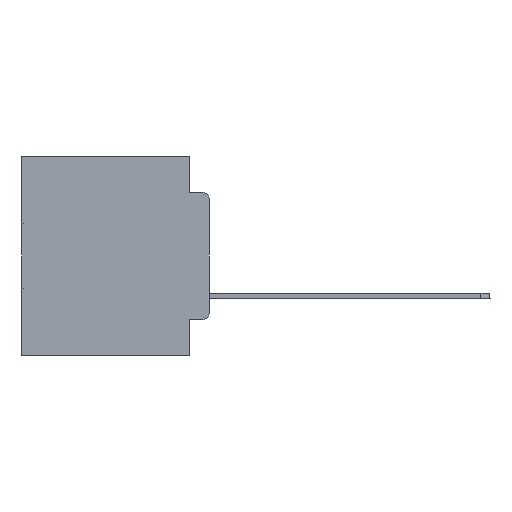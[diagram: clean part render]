
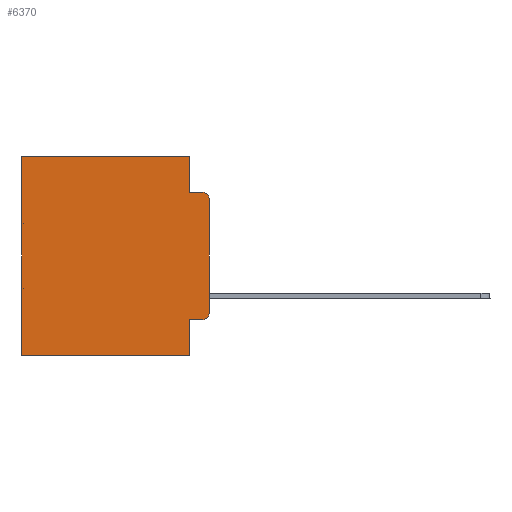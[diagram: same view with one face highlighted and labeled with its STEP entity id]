
A CAD part, left-side view. The second image highlights one B-rep face of the part: STEP entity #6370.
In plain terms, the highlighted planar face has unit normal (-1, 0, 0).
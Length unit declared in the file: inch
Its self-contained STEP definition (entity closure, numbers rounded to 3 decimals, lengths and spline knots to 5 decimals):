
#799 = EDGE_CURVE ( 'NONE', #15589, #9486, #19272, .T. ) ;
#1343 = CARTESIAN_POINT ( 'NONE',  ( 0.298, 0.473, 0. ) ) ;
#1909 = VERTEX_POINT ( 'NONE', #21501 ) ;
#2618 = CARTESIAN_POINT ( 'NONE',  ( 0.298, 0.051, -0.4115 ) ) ;
#3227 = PLANE ( 'NONE',  #21137 ) ;
#3861 = VERTEX_POINT ( 'NONE', #28291 ) ;
#4021 = EDGE_CURVE ( 'NONE', #1909, #19858, #5261, .T. ) ;
#4285 = DIRECTION ( 'NONE',  ( 0., 0., -1. ) ) ;
#5261 = LINE ( 'NONE', #8341, #31345 ) ;
#5583 = ORIENTED_EDGE ( 'NONE', *, *, #799, .F. ) ;
#6370 = ADVANCED_FACE ( 'NONE', ( #11471 ), #3227, .F. ) ;
#6376 = CARTESIAN_POINT ( 'NONE',  ( 0.298, 0., -0.1085 ) ) ;
#6698 = CARTESIAN_POINT ( 'NONE',  ( 0.298, 0.051, -0.5 ) ) ;
#6998 = VECTOR ( 'NONE', #26676, 39.37008 ) ;
#7429 = CARTESIAN_POINT ( 'NONE',  ( 0.298, 0.02, -0.3915 ) ) ;
#7465 = CIRCLE ( 'NONE', #21146, 0.02 ) ;
#7499 = CARTESIAN_POINT ( 'NONE',  ( 0.298, 0.02, -0.1085 ) ) ;
#7534 = DIRECTION ( 'NONE',  ( 0., 0., -1. ) ) ;
#7859 = LINE ( 'NONE', #16187, #13393 ) ;
#8133 = EDGE_CURVE ( 'NONE', #19858, #24229, #7859, .T. ) ;
#8341 = CARTESIAN_POINT ( 'NONE',  ( 0.298, 0., 0. ) ) ;
#8645 = DIRECTION ( 'NONE',  ( 0., 0., -1. ) ) ;
#9019 = CARTESIAN_POINT ( 'NONE',  ( 0.298, 0., -0.5 ) ) ;
#9377 = CARTESIAN_POINT ( 'NONE',  ( 0.298, 0.051, -0.0885 ) ) ;
#9486 = VERTEX_POINT ( 'NONE', #17530 ) ;
#9491 = CARTESIAN_POINT ( 'NONE',  ( 0.298, 0., 0. ) ) ;
#10018 = LINE ( 'NONE', #21835, #23842 ) ;
#10468 = VERTEX_POINT ( 'NONE', #26962 ) ;
#10809 = DIRECTION ( 'NONE',  ( 0., 0., -1. ) ) ;
#11471 = FACE_OUTER_BOUND ( 'NONE', #17562, .T. ) ;
#11542 = CARTESIAN_POINT ( 'NONE',  ( 0.298, 0.051, 0. ) ) ;
#12180 = VECTOR ( 'NONE', #17314, 39.37008 ) ;
#12218 = EDGE_CURVE ( 'NONE', #10468, #29105, #25719, .T. ) ;
#12295 = DIRECTION ( 'NONE',  ( -1., 0., 0. ) ) ;
#12555 = ORIENTED_EDGE ( 'NONE', *, *, #19096, .T. ) ;
#12607 = CIRCLE ( 'NONE', #27910, 0.02 ) ;
#13294 = CARTESIAN_POINT ( 'NONE',  ( 0.298, 0., 0. ) ) ;
#13310 = VERTEX_POINT ( 'NONE', #17510 ) ;
#13393 = VECTOR ( 'NONE', #10809, 39.37008 ) ;
#13462 = ORIENTED_EDGE ( 'NONE', *, *, #27746, .T. ) ;
#15589 = VERTEX_POINT ( 'NONE', #6376 ) ;
#16187 = CARTESIAN_POINT ( 'NONE',  ( 0.298, 0.473, 0. ) ) ;
#16481 = ORIENTED_EDGE ( 'NONE', *, *, #29356, .F. ) ;
#16874 = LINE ( 'NONE', #9019, #6998 ) ;
#17314 = DIRECTION ( 'NONE',  ( 0., 0., -1. ) ) ;
#17510 = CARTESIAN_POINT ( 'NONE',  ( 0.298, 0.02, -0.4115 ) ) ;
#17530 = CARTESIAN_POINT ( 'NONE',  ( 0.298, 0., -0.3915 ) ) ;
#17562 = EDGE_LOOP ( 'NONE', ( #5583, #30269, #29811, #16481, #19439, #17595, #25007, #20976, #12555, #13462 ) ) ;
#17595 = ORIENTED_EDGE ( 'NONE', *, *, #8133, .T. ) ;
#18787 = DIRECTION ( 'NONE',  ( 1., 0., 0. ) ) ;
#19096 = EDGE_CURVE ( 'NONE', #3861, #13310, #23813, .T. ) ;
#19272 = LINE ( 'NONE', #9491, #12180 ) ;
#19439 = ORIENTED_EDGE ( 'NONE', *, *, #4021, .T. ) ;
#19858 = VERTEX_POINT ( 'NONE', #1343 ) ;
#20429 = CARTESIAN_POINT ( 'NONE',  ( 0.298, 0.02, -0.0885 ) ) ;
#20976 = ORIENTED_EDGE ( 'NONE', *, *, #22104, .F. ) ;
#21137 = AXIS2_PLACEMENT_3D ( 'NONE', #13294, #18787, #23752 ) ;
#21146 = AXIS2_PLACEMENT_3D ( 'NONE', #7429, #12295, #7534 ) ;
#21501 = CARTESIAN_POINT ( 'NONE',  ( 0.298, 0.051, 0. ) ) ;
#21835 = CARTESIAN_POINT ( 'NONE',  ( 0.298, 0.051, 0. ) ) ;
#22104 = EDGE_CURVE ( 'NONE', #3861, #28813, #10018, .T. ) ;
#22504 = DIRECTION ( 'NONE',  ( 0., 0., -1. ) ) ;
#22786 = DIRECTION ( 'NONE',  ( 0., -1., 0. ) ) ;
#23182 = CARTESIAN_POINT ( 'NONE',  ( 0.298, 0.473, -0.5 ) ) ;
#23752 = DIRECTION ( 'NONE',  ( 0., 0., -1. ) ) ;
#23813 = LINE ( 'NONE', #2618, #26584 ) ;
#23842 = VECTOR ( 'NONE', #4285, 39.37008 ) ;
#24133 = VECTOR ( 'NONE', #32117, 39.37008 ) ;
#24229 = VERTEX_POINT ( 'NONE', #23182 ) ;
#24827 = EDGE_CURVE ( 'NONE', #15589, #29105, #12607, .T. ) ;
#25007 = ORIENTED_EDGE ( 'NONE', *, *, #28888, .F. ) ;
#25156 = DIRECTION ( 'NONE',  ( -1., 0., 0. ) ) ;
#25719 = LINE ( 'NONE', #9377, #24133 ) ;
#26221 = DIRECTION ( 'NONE',  ( 0., 1., 0. ) ) ;
#26584 = VECTOR ( 'NONE', #22786, 39.37008 ) ;
#26676 = DIRECTION ( 'NONE',  ( 0., 1., 0. ) ) ;
#26962 = CARTESIAN_POINT ( 'NONE',  ( 0.298, 0.051, -0.0885 ) ) ;
#27746 = EDGE_CURVE ( 'NONE', #13310, #9486, #7465, .T. ) ;
#27910 = AXIS2_PLACEMENT_3D ( 'NONE', #7499, #25156, #22504 ) ;
#28291 = CARTESIAN_POINT ( 'NONE',  ( 0.298, 0.051, -0.4115 ) ) ;
#28813 = VERTEX_POINT ( 'NONE', #6698 ) ;
#28888 = EDGE_CURVE ( 'NONE', #28813, #24229, #16874, .T. ) ;
#29105 = VERTEX_POINT ( 'NONE', #20429 ) ;
#29356 = EDGE_CURVE ( 'NONE', #1909, #10468, #30647, .T. ) ;
#29811 = ORIENTED_EDGE ( 'NONE', *, *, #12218, .F. ) ;
#30269 = ORIENTED_EDGE ( 'NONE', *, *, #24827, .T. ) ;
#30647 = LINE ( 'NONE', #11542, #31451 ) ;
#31345 = VECTOR ( 'NONE', #26221, 39.37008 ) ;
#31451 = VECTOR ( 'NONE', #8645, 39.37008 ) ;
#32117 = DIRECTION ( 'NONE',  ( 0., -1., 0. ) ) ;
